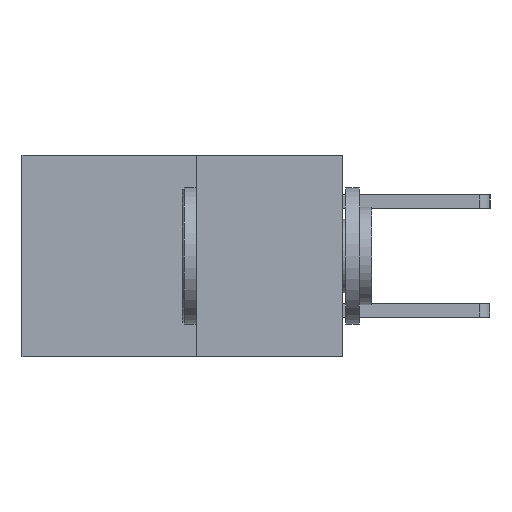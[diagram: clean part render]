
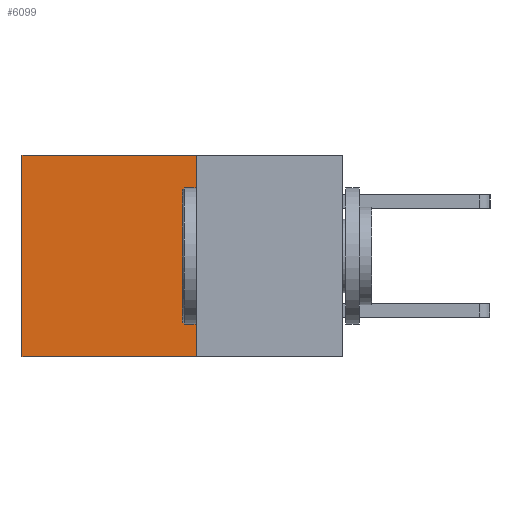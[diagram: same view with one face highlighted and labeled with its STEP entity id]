
A CAD part, left-side view. The second image highlights one B-rep face of the part: STEP entity #6099.
In plain terms, the highlighted planar face has unit normal (-1, 0, 0).
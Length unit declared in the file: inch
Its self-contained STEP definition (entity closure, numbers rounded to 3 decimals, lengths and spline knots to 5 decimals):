
#123 = CARTESIAN_POINT ( 'NONE',  ( 0.277, 0.27, -0.37 ) ) ;
#211 = CARTESIAN_POINT ( 'NONE',  ( 0.277, 0.59, 0. ) ) ;
#413 = ORIENTED_EDGE ( 'NONE', *, *, #414, .F. ) ;
#414 = EDGE_CURVE ( 'NONE', #6546, #2868, #10605, .T. ) ;
#761 = ORIENTED_EDGE ( 'NONE', *, *, #1412, .T. ) ;
#900 = DIRECTION ( 'NONE',  ( 1., 0., 0. ) ) ;
#985 = DIRECTION ( 'NONE',  ( 0., 0., -1. ) ) ;
#1412 = EDGE_CURVE ( 'NONE', #9237, #10171, #7290, .T. ) ;
#1492 = CARTESIAN_POINT ( 'NONE',  ( 0.277, 0.59, -0.37 ) ) ;
#1571 = DIRECTION ( 'NONE',  ( 0., 1., 0. ) ) ;
#1615 = EDGE_CURVE ( 'NONE', #10171, #2868, #7725, .T. ) ;
#2461 = CARTESIAN_POINT ( 'NONE',  ( 0.277, 0.27, 0. ) ) ;
#2478 = LINE ( 'NONE', #3421, #12250 ) ;
#2808 = FACE_OUTER_BOUND ( 'NONE', #5106, .T. ) ;
#2868 = VERTEX_POINT ( 'NONE', #8823 ) ;
#3115 = CARTESIAN_POINT ( 'NONE',  ( 0.277, 0.27, 0. ) ) ;
#3190 = ORIENTED_EDGE ( 'NONE', *, *, #5029, .F. ) ;
#3421 = CARTESIAN_POINT ( 'NONE',  ( 0.277, 0.27, -0.37 ) ) ;
#3892 = CARTESIAN_POINT ( 'NONE',  ( 0.277, 0.27, -0.37 ) ) ;
#5029 = EDGE_CURVE ( 'NONE', #9237, #6546, #2478, .T. ) ;
#5106 = EDGE_LOOP ( 'NONE', ( #7738, #413, #3190, #761 ) ) ;
#5373 = DIRECTION ( 'NONE',  ( 0., 0., -1. ) ) ;
#5854 = PLANE ( 'NONE',  #6397 ) ;
#6099 = ADVANCED_FACE ( 'NONE', ( #2808 ), #5854, .F. ) ;
#6397 = AXIS2_PLACEMENT_3D ( 'NONE', #3892, #900, #7813 ) ;
#6546 = VERTEX_POINT ( 'NONE', #10218 ) ;
#7290 = LINE ( 'NONE', #2461, #11907 ) ;
#7725 = LINE ( 'NONE', #1492, #12331 ) ;
#7738 = ORIENTED_EDGE ( 'NONE', *, *, #1615, .T. ) ;
#7813 = DIRECTION ( 'NONE',  ( 0., 0., -1. ) ) ;
#7843 = VECTOR ( 'NONE', #9882, 39.37008 ) ;
#8823 = CARTESIAN_POINT ( 'NONE',  ( 0.277, 0.59, -0.37 ) ) ;
#9237 = VERTEX_POINT ( 'NONE', #3115 ) ;
#9882 = DIRECTION ( 'NONE',  ( 0., 1., 0. ) ) ;
#10171 = VERTEX_POINT ( 'NONE', #211 ) ;
#10218 = CARTESIAN_POINT ( 'NONE',  ( 0.277, 0.27, -0.37 ) ) ;
#10605 = LINE ( 'NONE', #123, #7843 ) ;
#11907 = VECTOR ( 'NONE', #1571, 39.37008 ) ;
#12250 = VECTOR ( 'NONE', #5373, 39.37008 ) ;
#12331 = VECTOR ( 'NONE', #985, 39.37008 ) ;
